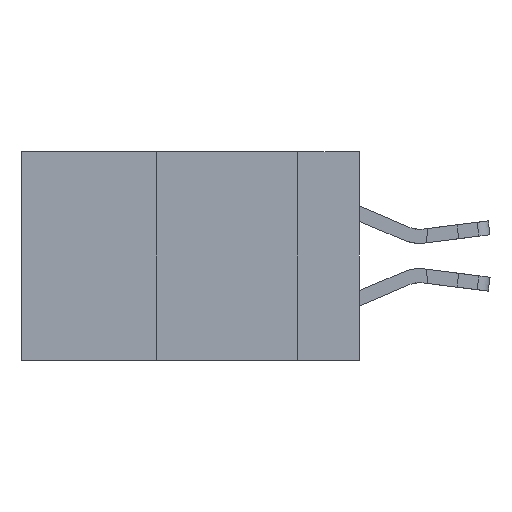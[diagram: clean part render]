
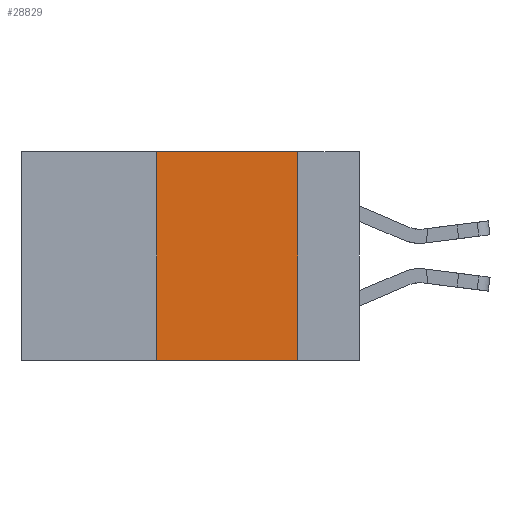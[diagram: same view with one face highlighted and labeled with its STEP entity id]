
A CAD part, left-side view. The second image highlights one B-rep face of the part: STEP entity #28829.
In plain terms, the highlighted planar face has unit normal (-1, 0, 0).
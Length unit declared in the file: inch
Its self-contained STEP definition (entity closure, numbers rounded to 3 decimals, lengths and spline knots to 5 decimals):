
#541 = LINE ( 'NONE', #21240, #20485 ) ;
#1805 = FACE_OUTER_BOUND ( 'NONE', #29306, .T. ) ;
#3285 = EDGE_CURVE ( 'NONE', #30884, #27349, #32112, .T. ) ;
#6747 = CARTESIAN_POINT ( 'NONE',  ( 0., 0.36, -0.37 ) ) ;
#7679 = CARTESIAN_POINT ( 'NONE',  ( 0., 0.36, 0. ) ) ;
#8144 = DIRECTION ( 'NONE',  ( 0., -1., 0. ) ) ;
#8685 = CARTESIAN_POINT ( 'NONE',  ( 0., 0.36, 0. ) ) ;
#8716 = ORIENTED_EDGE ( 'NONE', *, *, #18192, .F. ) ;
#8968 = VECTOR ( 'NONE', #13012, 39.37008 ) ;
#10170 = VERTEX_POINT ( 'NONE', #27567 ) ;
#10193 = CARTESIAN_POINT ( 'NONE',  ( 0., 0.6, 0. ) ) ;
#12756 = DIRECTION ( 'NONE',  ( 0., 0., -1. ) ) ;
#13012 = DIRECTION ( 'NONE',  ( 0., 0., 1. ) ) ;
#14834 = VERTEX_POINT ( 'NONE', #8685 ) ;
#16537 = DIRECTION ( 'NONE',  ( 0., -1., 0. ) ) ;
#17865 = PLANE ( 'NONE',  #19410 ) ;
#18055 = LINE ( 'NONE', #31752, #33102 ) ;
#18192 = EDGE_CURVE ( 'NONE', #10170, #27349, #541, .T. ) ;
#18853 = ORIENTED_EDGE ( 'NONE', *, *, #3285, .T. ) ;
#19410 = AXIS2_PLACEMENT_3D ( 'NONE', #10193, #28124, #12756 ) ;
#20485 = VECTOR ( 'NONE', #26354, 39.37008 ) ;
#21088 = LINE ( 'NONE', #7679, #8968 ) ;
#21240 = CARTESIAN_POINT ( 'NONE',  ( 0., 0.11, 0. ) ) ;
#24063 = EDGE_CURVE ( 'NONE', #30884, #14834, #21088, .T. ) ;
#26354 = DIRECTION ( 'NONE',  ( 0., 0., -1. ) ) ;
#27349 = VERTEX_POINT ( 'NONE', #30906 ) ;
#27567 = CARTESIAN_POINT ( 'NONE',  ( 0., 0.11, 0. ) ) ;
#28124 = DIRECTION ( 'NONE',  ( 1., 0., 0. ) ) ;
#28465 = EDGE_CURVE ( 'NONE', #14834, #10170, #18055, .T. ) ;
#28829 = ADVANCED_FACE ( 'NONE', ( #1805 ), #17865, .F. ) ;
#29306 = EDGE_LOOP ( 'NONE', ( #8716, #29984, #31538, #18853 ) ) ;
#29984 = ORIENTED_EDGE ( 'NONE', *, *, #28465, .F. ) ;
#30884 = VERTEX_POINT ( 'NONE', #6747 ) ;
#30906 = CARTESIAN_POINT ( 'NONE',  ( 0., 0.11, -0.37 ) ) ;
#31220 = CARTESIAN_POINT ( 'NONE',  ( 0., 0.6, -0.37 ) ) ;
#31538 = ORIENTED_EDGE ( 'NONE', *, *, #24063, .F. ) ;
#31752 = CARTESIAN_POINT ( 'NONE',  ( 0., 0.6, 0. ) ) ;
#32112 = LINE ( 'NONE', #31220, #32898 ) ;
#32898 = VECTOR ( 'NONE', #8144, 39.37008 ) ;
#33102 = VECTOR ( 'NONE', #16537, 39.37008 ) ;
